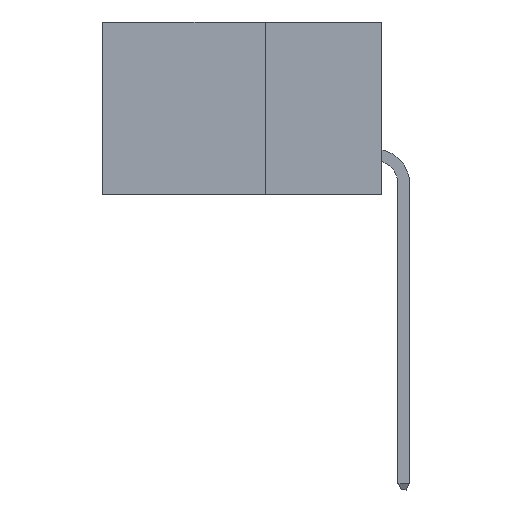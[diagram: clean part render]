
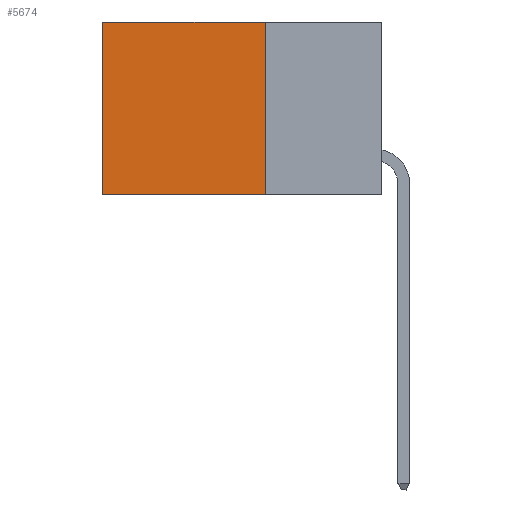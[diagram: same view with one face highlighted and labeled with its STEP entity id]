
A CAD part, left-side view. The second image highlights one B-rep face of the part: STEP entity #5674.
In plain terms, the highlighted planar face has unit normal (-1, 0, 0).
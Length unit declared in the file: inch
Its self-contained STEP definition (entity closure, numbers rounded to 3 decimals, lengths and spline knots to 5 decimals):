
#1087 = DIRECTION ( 'NONE',  ( 0., 0., -1. ) ) ;
#1839 = VERTEX_POINT ( 'NONE', #13772 ) ;
#1985 = PLANE ( 'NONE',  #5950 ) ;
#2091 = VECTOR ( 'NONE', #1087, 39.37008 ) ;
#2483 = CARTESIAN_POINT ( 'NONE',  ( 0.2875, 0.25, -0.37 ) ) ;
#2848 = CARTESIAN_POINT ( 'NONE',  ( 0.2875, 0.6, 0. ) ) ;
#2991 = DIRECTION ( 'NONE',  ( 0., 0., -1. ) ) ;
#3420 = VERTEX_POINT ( 'NONE', #10086 ) ;
#3514 = VECTOR ( 'NONE', #6771, 39.37008 ) ;
#3753 = LINE ( 'NONE', #6834, #3514 ) ;
#4059 = CARTESIAN_POINT ( 'NONE',  ( 0.2875, 0.25, 0. ) ) ;
#4315 = LINE ( 'NONE', #13017, #2091 ) ;
#5213 = FACE_OUTER_BOUND ( 'NONE', #9996, .T. ) ;
#5632 = LINE ( 'NONE', #6062, #9855 ) ;
#5674 = ADVANCED_FACE ( 'NONE', ( #5213 ), #1985, .F. ) ;
#5950 = AXIS2_PLACEMENT_3D ( 'NONE', #4059, #12910, #2991 ) ;
#6062 = CARTESIAN_POINT ( 'NONE',  ( 0.2875, 0.25, 0. ) ) ;
#6561 = VERTEX_POINT ( 'NONE', #2848 ) ;
#6771 = DIRECTION ( 'NONE',  ( 0., 0., -1. ) ) ;
#6834 = CARTESIAN_POINT ( 'NONE',  ( 0.2875, 0.25, 0. ) ) ;
#7781 = EDGE_CURVE ( 'NONE', #3420, #1839, #12331, .T. ) ;
#8268 = DIRECTION ( 'NONE',  ( 0., 1., 0. ) ) ;
#8474 = EDGE_CURVE ( 'NONE', #6561, #1839, #4315, .T. ) ;
#8657 = ORIENTED_EDGE ( 'NONE', *, *, #9874, .F. ) ;
#9840 = ORIENTED_EDGE ( 'NONE', *, *, #10564, .T. ) ;
#9855 = VECTOR ( 'NONE', #8268, 39.37008 ) ;
#9874 = EDGE_CURVE ( 'NONE', #11207, #3420, #3753, .T. ) ;
#9967 = VECTOR ( 'NONE', #11263, 39.37008 ) ;
#9972 = CARTESIAN_POINT ( 'NONE',  ( 0.2875, 0.25, 0. ) ) ;
#9996 = EDGE_LOOP ( 'NONE', ( #12888, #12157, #8657, #9840 ) ) ;
#10086 = CARTESIAN_POINT ( 'NONE',  ( 0.2875, 0.25, -0.37 ) ) ;
#10564 = EDGE_CURVE ( 'NONE', #11207, #6561, #5632, .T. ) ;
#11207 = VERTEX_POINT ( 'NONE', #9972 ) ;
#11263 = DIRECTION ( 'NONE',  ( 0., 1., 0. ) ) ;
#12157 = ORIENTED_EDGE ( 'NONE', *, *, #7781, .F. ) ;
#12331 = LINE ( 'NONE', #2483, #9967 ) ;
#12888 = ORIENTED_EDGE ( 'NONE', *, *, #8474, .T. ) ;
#12910 = DIRECTION ( 'NONE',  ( 1., 0., 0. ) ) ;
#13017 = CARTESIAN_POINT ( 'NONE',  ( 0.2875, 0.6, 0. ) ) ;
#13772 = CARTESIAN_POINT ( 'NONE',  ( 0.2875, 0.6, -0.37 ) ) ;
